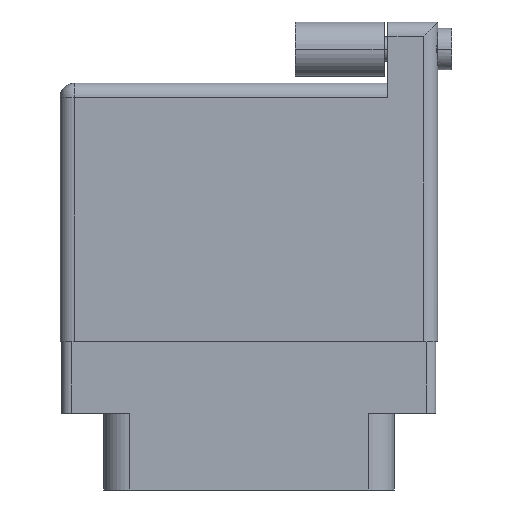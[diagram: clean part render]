
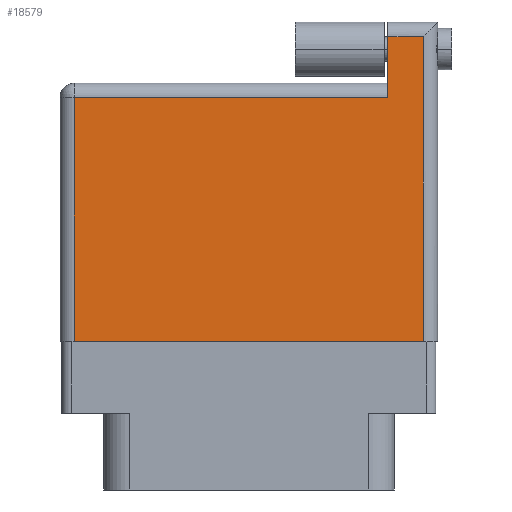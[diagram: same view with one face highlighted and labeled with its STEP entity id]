
A CAD part, front view. The second image highlights one B-rep face of the part: STEP entity #18579.
In plain terms, the highlighted face is planar.
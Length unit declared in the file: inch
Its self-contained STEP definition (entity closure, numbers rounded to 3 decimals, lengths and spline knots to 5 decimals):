
#1082 = PLANE ( 'NONE',  #17220 ) ;
#2703 = VERTEX_POINT ( 'NONE', #10114 ) ;
#3109 = DIRECTION ( 'NONE',  ( -1., 0., 0. ) ) ;
#3487 = ORIENTED_EDGE ( 'NONE', *, *, #23135, .T. ) ;
#3596 = VERTEX_POINT ( 'NONE', #14654 ) ;
#3922 = CARTESIAN_POINT ( 'NONE',  ( 1.15, 1.12, 0. ) ) ;
#4197 = VECTOR ( 'NONE', #3109, 39.37008 ) ;
#4532 = ORIENTED_EDGE ( 'NONE', *, *, #12061, .T. ) ;
#4990 = ORIENTED_EDGE ( 'NONE', *, *, #23055, .T. ) ;
#5456 = LINE ( 'NONE', #11155, #14794 ) ;
#5499 = CARTESIAN_POINT ( 'NONE',  ( 0.05, 0., 0. ) ) ;
#5896 = CARTESIAN_POINT ( 'NONE',  ( 1.275, 1.07, 0. ) ) ;
#6023 = EDGE_LOOP ( 'NONE', ( #4990, #3487, #14807, #12015, #8329, #4532 ) ) ;
#6915 = LINE ( 'NONE', #3922, #7182 ) ;
#7029 = CARTESIAN_POINT ( 'NONE',  ( 0., 0.906, 0. ) ) ;
#7033 = LINE ( 'NONE', #21130, #4197 ) ;
#7182 = VECTOR ( 'NONE', #16474, 39.37008 ) ;
#8329 = ORIENTED_EDGE ( 'NONE', *, *, #21593, .T. ) ;
#9367 = VERTEX_POINT ( 'NONE', #21705 ) ;
#9811 = VECTOR ( 'NONE', #12933, 39.37008 ) ;
#9834 = LINE ( 'NONE', #11560, #21352 ) ;
#10114 = CARTESIAN_POINT ( 'NONE',  ( 0.05, 0., 0. ) ) ;
#11155 = CARTESIAN_POINT ( 'NONE',  ( 0., 0., 0. ) ) ;
#11481 = VERTEX_POINT ( 'NONE', #16491 ) ;
#11560 = CARTESIAN_POINT ( 'NONE',  ( 0., 1.07, 0. ) ) ;
#12015 = ORIENTED_EDGE ( 'NONE', *, *, #17493, .T. ) ;
#12061 = EDGE_CURVE ( 'NONE', #20183, #2703, #21613, .T. ) ;
#12933 = DIRECTION ( 'NONE',  ( 0., -1., 0. ) ) ;
#14654 = CARTESIAN_POINT ( 'NONE',  ( 1.275, 0., 0. ) ) ;
#14763 = LINE ( 'NONE', #15270, #17609 ) ;
#14794 = VECTOR ( 'NONE', #20130, 39.37008 ) ;
#14807 = ORIENTED_EDGE ( 'NONE', *, *, #16113, .T. ) ;
#15270 = CARTESIAN_POINT ( 'NONE',  ( 1.275, 1.12, 0. ) ) ;
#16113 = EDGE_CURVE ( 'NONE', #17594, #11481, #9834, .T. ) ;
#16474 = DIRECTION ( 'NONE',  ( 0., -1., 0. ) ) ;
#16491 = CARTESIAN_POINT ( 'NONE',  ( 1.15, 1.07, 0. ) ) ;
#17220 = AXIS2_PLACEMENT_3D ( 'NONE', #7029, #23244, #19657 ) ;
#17493 = EDGE_CURVE ( 'NONE', #11481, #9367, #6915, .T. ) ;
#17594 = VERTEX_POINT ( 'NONE', #5896 ) ;
#17609 = VECTOR ( 'NONE', #18743, 39.37008 ) ;
#18579 = ADVANCED_FACE ( 'NONE', ( #20389 ), #1082, .F. ) ;
#18743 = DIRECTION ( 'NONE',  ( 0., 1., 0. ) ) ;
#18893 = DIRECTION ( 'NONE',  ( -1., 0., 0. ) ) ;
#19657 = DIRECTION ( 'NONE',  ( -1., 0., 0. ) ) ;
#20130 = DIRECTION ( 'NONE',  ( 1., 0., 0. ) ) ;
#20183 = VERTEX_POINT ( 'NONE', #22707 ) ;
#20389 = FACE_OUTER_BOUND ( 'NONE', #6023, .T. ) ;
#21130 = CARTESIAN_POINT ( 'NONE',  ( 0., 0.856, 0. ) ) ;
#21352 = VECTOR ( 'NONE', #18893, 39.37008 ) ;
#21593 = EDGE_CURVE ( 'NONE', #9367, #20183, #7033, .T. ) ;
#21613 = LINE ( 'NONE', #5499, #9811 ) ;
#21705 = CARTESIAN_POINT ( 'NONE',  ( 1.15, 0.856, 0. ) ) ;
#22707 = CARTESIAN_POINT ( 'NONE',  ( 0.05, 0.856, 0. ) ) ;
#23055 = EDGE_CURVE ( 'NONE', #2703, #3596, #5456, .T. ) ;
#23135 = EDGE_CURVE ( 'NONE', #3596, #17594, #14763, .T. ) ;
#23244 = DIRECTION ( 'NONE',  ( 0., 0., -1. ) ) ;
